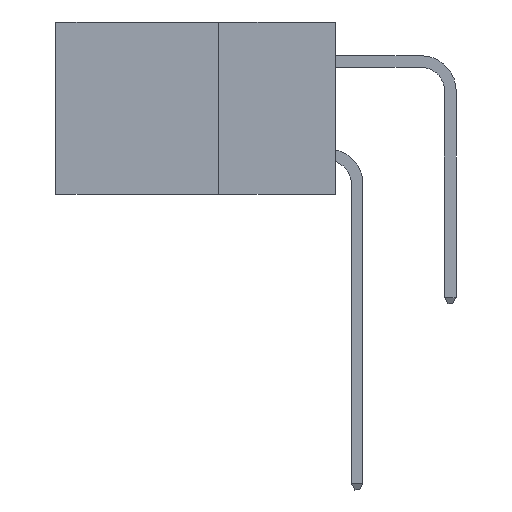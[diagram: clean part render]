
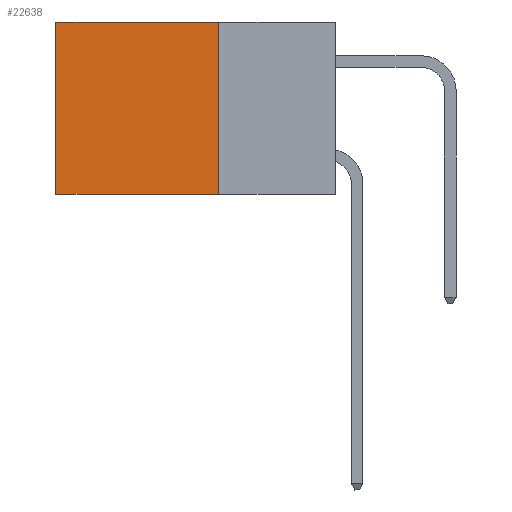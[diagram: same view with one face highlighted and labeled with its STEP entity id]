
A CAD part, left-side view. The second image highlights one B-rep face of the part: STEP entity #22638.
In plain terms, the highlighted planar face has unit normal (-1, 0, 0).
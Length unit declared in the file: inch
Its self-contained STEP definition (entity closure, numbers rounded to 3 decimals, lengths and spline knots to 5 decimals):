
#503 = CARTESIAN_POINT ( 'NONE',  ( 0.2875, 0.25, 0. ) ) ;
#736 = DIRECTION ( 'NONE',  ( 1., 0., 0. ) ) ;
#1621 = ORIENTED_EDGE ( 'NONE', *, *, #2416, .F. ) ;
#2315 = VECTOR ( 'NONE', #26523, 39.37008 ) ;
#2416 = EDGE_CURVE ( 'NONE', #17454, #5493, #26228, .T. ) ;
#2488 = ORIENTED_EDGE ( 'NONE', *, *, #5185, .T. ) ;
#2499 = VECTOR ( 'NONE', #4869, 39.37008 ) ;
#2577 = CARTESIAN_POINT ( 'NONE',  ( 0.2875, 0.25, 0. ) ) ;
#2931 = DIRECTION ( 'NONE',  ( 0., 0., -1. ) ) ;
#4173 = LINE ( 'NONE', #6780, #2499 ) ;
#4750 = PLANE ( 'NONE',  #9933 ) ;
#4869 = DIRECTION ( 'NONE',  ( 0., 1., 0. ) ) ;
#5117 = LINE ( 'NONE', #13605, #26221 ) ;
#5185 = EDGE_CURVE ( 'NONE', #17454, #8716, #19012, .T. ) ;
#5493 = VERTEX_POINT ( 'NONE', #18474 ) ;
#6308 = CARTESIAN_POINT ( 'NONE',  ( 0.2875, 0.6, -0.37 ) ) ;
#6339 = CARTESIAN_POINT ( 'NONE',  ( 0.2875, 0.6, 0. ) ) ;
#6780 = CARTESIAN_POINT ( 'NONE',  ( 0.2875, 0.25, -0.37 ) ) ;
#7697 = EDGE_CURVE ( 'NONE', #8716, #12275, #5117, .T. ) ;
#8716 = VERTEX_POINT ( 'NONE', #6339 ) ;
#9933 = AXIS2_PLACEMENT_3D ( 'NONE', #21623, #736, #2931 ) ;
#11662 = EDGE_LOOP ( 'NONE', ( #15102, #18866, #1621, #2488 ) ) ;
#12275 = VERTEX_POINT ( 'NONE', #6308 ) ;
#13605 = CARTESIAN_POINT ( 'NONE',  ( 0.2875, 0.6, 0. ) ) ;
#15102 = ORIENTED_EDGE ( 'NONE', *, *, #7697, .T. ) ;
#15269 = DIRECTION ( 'NONE',  ( 0., 0., -1. ) ) ;
#17454 = VERTEX_POINT ( 'NONE', #503 ) ;
#18474 = CARTESIAN_POINT ( 'NONE',  ( 0.2875, 0.25, -0.37 ) ) ;
#18857 = FACE_OUTER_BOUND ( 'NONE', #11662, .T. ) ;
#18866 = ORIENTED_EDGE ( 'NONE', *, *, #18968, .F. ) ;
#18968 = EDGE_CURVE ( 'NONE', #5493, #12275, #4173, .T. ) ;
#19012 = LINE ( 'NONE', #24256, #2315 ) ;
#19861 = DIRECTION ( 'NONE',  ( 0., 0., -1. ) ) ;
#21623 = CARTESIAN_POINT ( 'NONE',  ( 0.2875, 0.25, 0. ) ) ;
#21860 = VECTOR ( 'NONE', #15269, 39.37008 ) ;
#22638 = ADVANCED_FACE ( 'NONE', ( #18857 ), #4750, .F. ) ;
#24256 = CARTESIAN_POINT ( 'NONE',  ( 0.2875, 0.25, 0. ) ) ;
#26221 = VECTOR ( 'NONE', #19861, 39.37008 ) ;
#26228 = LINE ( 'NONE', #2577, #21860 ) ;
#26523 = DIRECTION ( 'NONE',  ( 0., 1., 0. ) ) ;
